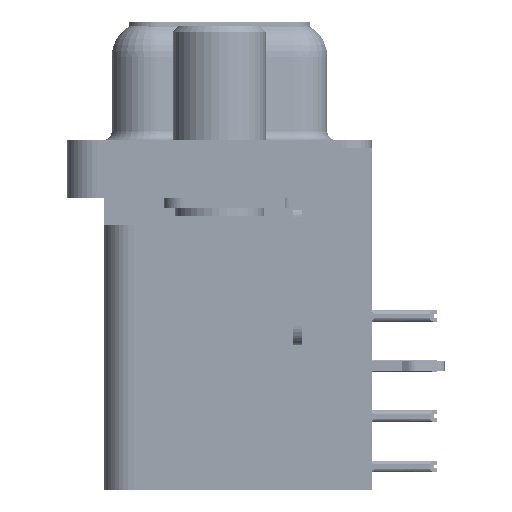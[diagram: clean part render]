
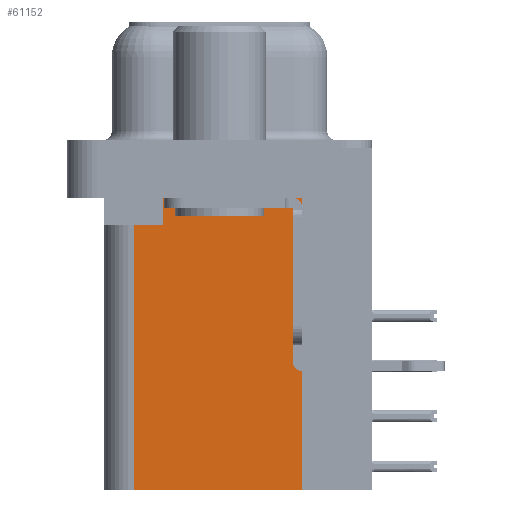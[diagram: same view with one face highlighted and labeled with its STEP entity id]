
A CAD part, left-side view. The second image highlights one B-rep face of the part: STEP entity #61152.
In plain terms, the highlighted planar face has unit normal (-1, 0, 0).
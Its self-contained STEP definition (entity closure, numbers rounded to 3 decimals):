
#849 = VERTEX_POINT ( 'NONE', #12925 ) ;
#2032 = CARTESIAN_POINT ( 'NONE',  ( 3.75, -4.2, -17.3 ) ) ;
#2145 = VERTEX_POINT ( 'NONE', #2032 ) ;
#2423 = VECTOR ( 'NONE', #44832, 1000. ) ;
#6337 = CARTESIAN_POINT ( 'NONE',  ( 3.75, -4.2, -2.5 ) ) ;
#8046 = ORIENTED_EDGE ( 'NONE', *, *, #64082, .T. ) ;
#9673 = FACE_OUTER_BOUND ( 'NONE', #34979, .T. ) ;
#10634 = DIRECTION ( 'NONE',  ( 0., 1., 0. ) ) ;
#12506 = ORIENTED_EDGE ( 'NONE', *, *, #68616, .T. ) ;
#12579 = LINE ( 'NONE', #22133, #69647 ) ;
#12925 = CARTESIAN_POINT ( 'NONE',  ( 3.75, 2.85, -2.5 ) ) ;
#17412 = LINE ( 'NONE', #17644, #58054 ) ;
#17644 = CARTESIAN_POINT ( 'NONE',  ( 3.75, -4.2, -17.3 ) ) ;
#18004 = EDGE_CURVE ( 'NONE', #50392, #849, #18538, .T. ) ;
#18538 = LINE ( 'NONE', #38168, #60960 ) ;
#19478 = ORIENTED_EDGE ( 'NONE', *, *, #32351, .F. ) ;
#19629 = DIRECTION ( 'NONE',  ( 0., 0., -1. ) ) ;
#21397 = VECTOR ( 'NONE', #64250, 1000. ) ;
#22133 = CARTESIAN_POINT ( 'NONE',  ( 3.75, -4.2, -17.3 ) ) ;
#22834 = EDGE_CURVE ( 'NONE', #24891, #44417, #31753, .T. ) ;
#23173 = DIRECTION ( 'NONE',  ( 0., 1., 0. ) ) ;
#23298 = CARTESIAN_POINT ( 'NONE',  ( 3.75, -4.2, -17.3 ) ) ;
#24891 = VERTEX_POINT ( 'NONE', #26970 ) ;
#25530 = CARTESIAN_POINT ( 'NONE',  ( 3.75, 0., -3.9 ) ) ;
#26970 = CARTESIAN_POINT ( 'NONE',  ( 3.75, 4.35, -17.3 ) ) ;
#28830 = DIRECTION ( 'NONE',  ( 0., 1., 0. ) ) ;
#31753 = LINE ( 'NONE', #39223, #2423 ) ;
#32351 = EDGE_CURVE ( 'NONE', #2145, #24891, #17412, .T. ) ;
#34979 = EDGE_LOOP ( 'NONE', ( #40167, #8046, #42667, #70260, #19478, #12506 ) ) ;
#38168 = CARTESIAN_POINT ( 'NONE',  ( 3.75, -4.2, -2.5 ) ) ;
#39223 = CARTESIAN_POINT ( 'NONE',  ( 3.75, 4.35, -17.3 ) ) ;
#39643 = VERTEX_POINT ( 'NONE', #49536 ) ;
#40167 = ORIENTED_EDGE ( 'NONE', *, *, #18004, .T. ) ;
#42667 = ORIENTED_EDGE ( 'NONE', *, *, #57482, .T. ) ;
#43305 = CARTESIAN_POINT ( 'NONE',  ( 3.75, 4.35, -3.9 ) ) ;
#44417 = VERTEX_POINT ( 'NONE', #43305 ) ;
#44832 = DIRECTION ( 'NONE',  ( 0., 0., 1. ) ) ;
#48628 = LINE ( 'NONE', #52755, #65036 ) ;
#49498 = AXIS2_PLACEMENT_3D ( 'NONE', #23298, #62005, #28830 ) ;
#49536 = CARTESIAN_POINT ( 'NONE',  ( 3.75, 2.85, -3.9 ) ) ;
#50392 = VERTEX_POINT ( 'NONE', #6337 ) ;
#52755 = CARTESIAN_POINT ( 'NONE',  ( 3.75, 2.85, -3.9 ) ) ;
#56481 = PLANE ( 'NONE',  #49498 ) ;
#57482 = EDGE_CURVE ( 'NONE', #39643, #44417, #63757, .T. ) ;
#58054 = VECTOR ( 'NONE', #23173, 1000. ) ;
#60960 = VECTOR ( 'NONE', #10634, 1000. ) ;
#61152 = ADVANCED_FACE ( 'NONE', ( #9673 ), #56481, .F. ) ;
#62005 = DIRECTION ( 'NONE',  ( 1., 0., 0. ) ) ;
#63757 = LINE ( 'NONE', #25530, #21397 ) ;
#64082 = EDGE_CURVE ( 'NONE', #849, #39643, #48628, .T. ) ;
#64250 = DIRECTION ( 'NONE',  ( 0., 1., 0. ) ) ;
#65036 = VECTOR ( 'NONE', #19629, 1000. ) ;
#66333 = DIRECTION ( 'NONE',  ( 0., 0., 1. ) ) ;
#68616 = EDGE_CURVE ( 'NONE', #2145, #50392, #12579, .T. ) ;
#69647 = VECTOR ( 'NONE', #66333, 1000. ) ;
#70260 = ORIENTED_EDGE ( 'NONE', *, *, #22834, .F. ) ;
